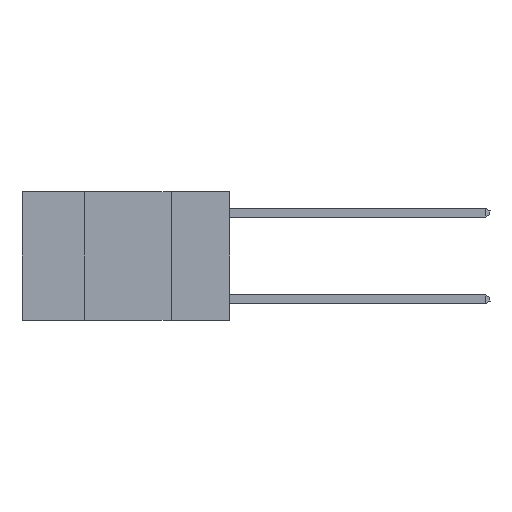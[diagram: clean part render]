
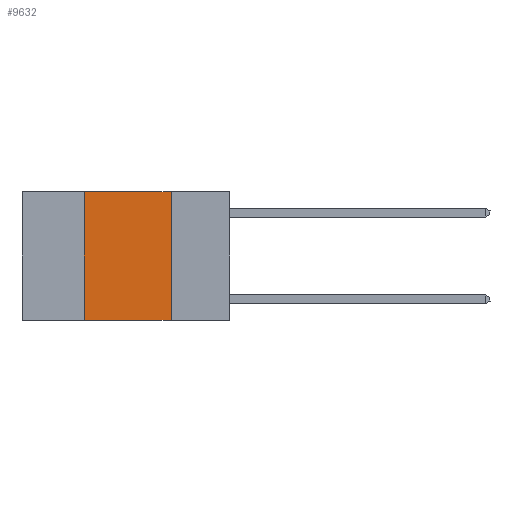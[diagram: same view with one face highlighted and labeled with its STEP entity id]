
A CAD part, left-side view. The second image highlights one B-rep face of the part: STEP entity #9632.
In plain terms, the highlighted planar face has unit normal (-1, 0, 0).
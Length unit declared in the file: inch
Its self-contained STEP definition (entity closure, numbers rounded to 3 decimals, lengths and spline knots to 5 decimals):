
#786 = VECTOR ( 'NONE', #13316, 39.37008 ) ;
#2013 = CARTESIAN_POINT ( 'NONE',  ( 0., 0.42, 0. ) ) ;
#2480 = CARTESIAN_POINT ( 'NONE',  ( 0., 0.42, -0.37 ) ) ;
#2545 = ORIENTED_EDGE ( 'NONE', *, *, #5592, .F. ) ;
#3127 = CARTESIAN_POINT ( 'NONE',  ( 0., 0.17, -0.37 ) ) ;
#3851 = LINE ( 'NONE', #8195, #12073 ) ;
#4147 = CARTESIAN_POINT ( 'NONE',  ( 0., 0.17, 0. ) ) ;
#4520 = EDGE_CURVE ( 'NONE', #13370, #6952, #7045, .T. ) ;
#4629 = LINE ( 'NONE', #8851, #786 ) ;
#4917 = DIRECTION ( 'NONE',  ( 1., 0., 0. ) ) ;
#4998 = ORIENTED_EDGE ( 'NONE', *, *, #4520, .T. ) ;
#5034 = VERTEX_POINT ( 'NONE', #2013 ) ;
#5592 = EDGE_CURVE ( 'NONE', #13370, #5034, #4629, .T. ) ;
#5669 = ORIENTED_EDGE ( 'NONE', *, *, #5819, .F. ) ;
#5819 = EDGE_CURVE ( 'NONE', #5034, #12217, #3851, .T. ) ;
#6952 = VERTEX_POINT ( 'NONE', #3127 ) ;
#7045 = LINE ( 'NONE', #11523, #13209 ) ;
#7067 = DIRECTION ( 'NONE',  ( 0., 0., -1. ) ) ;
#7217 = LINE ( 'NONE', #12545, #13708 ) ;
#8195 = CARTESIAN_POINT ( 'NONE',  ( 0., 0.6, 0. ) ) ;
#8851 = CARTESIAN_POINT ( 'NONE',  ( 0., 0.42, 0. ) ) ;
#9151 = ORIENTED_EDGE ( 'NONE', *, *, #9188, .F. ) ;
#9188 = EDGE_CURVE ( 'NONE', #12217, #6952, #7217, .T. ) ;
#9326 = FACE_OUTER_BOUND ( 'NONE', #9400, .T. ) ;
#9400 = EDGE_LOOP ( 'NONE', ( #9151, #5669, #2545, #4998 ) ) ;
#9632 = ADVANCED_FACE ( 'NONE', ( #9326 ), #10538, .F. ) ;
#10076 = AXIS2_PLACEMENT_3D ( 'NONE', #12453, #4917, #12529 ) ;
#10538 = PLANE ( 'NONE',  #10076 ) ;
#11376 = DIRECTION ( 'NONE',  ( 0., -1., 0. ) ) ;
#11523 = CARTESIAN_POINT ( 'NONE',  ( 0., 0.6, -0.37 ) ) ;
#12073 = VECTOR ( 'NONE', #13945, 39.37008 ) ;
#12217 = VERTEX_POINT ( 'NONE', #4147 ) ;
#12453 = CARTESIAN_POINT ( 'NONE',  ( 0., 0.6, 0. ) ) ;
#12529 = DIRECTION ( 'NONE',  ( 0., 0., -1. ) ) ;
#12545 = CARTESIAN_POINT ( 'NONE',  ( 0., 0.17, 0. ) ) ;
#13209 = VECTOR ( 'NONE', #11376, 39.37008 ) ;
#13316 = DIRECTION ( 'NONE',  ( 0., 0., 1. ) ) ;
#13370 = VERTEX_POINT ( 'NONE', #2480 ) ;
#13708 = VECTOR ( 'NONE', #7067, 39.37008 ) ;
#13945 = DIRECTION ( 'NONE',  ( 0., -1., 0. ) ) ;
